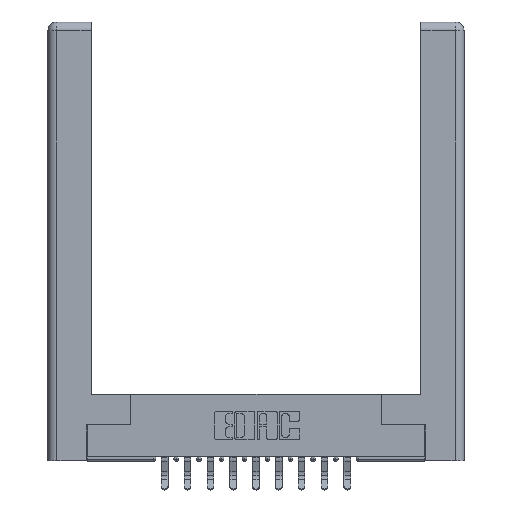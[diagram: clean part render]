
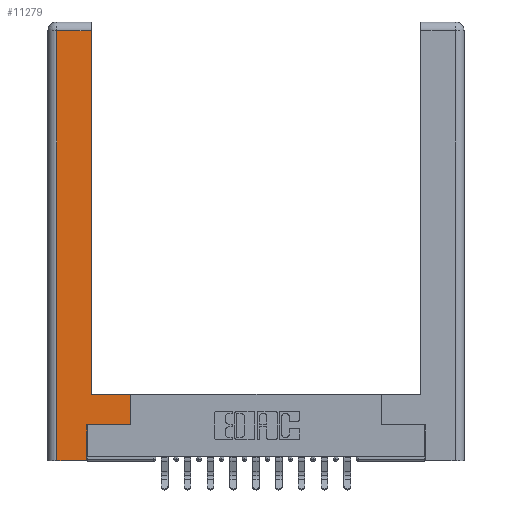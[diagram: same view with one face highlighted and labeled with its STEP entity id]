
A CAD part, top view. The second image highlights one B-rep face of the part: STEP entity #11279.
In plain terms, the highlighted planar face has unit normal (0, 0, 1).
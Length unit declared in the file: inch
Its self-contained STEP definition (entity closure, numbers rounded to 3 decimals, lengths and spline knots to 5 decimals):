
#179 = AXIS2_PLACEMENT_3D ( 'NONE', #3150, #12336, #1984 ) ;
#223 = VERTEX_POINT ( 'NONE', #7931 ) ;
#226 = LINE ( 'NONE', #12512, #13695 ) ;
#437 = ORIENTED_EDGE ( 'NONE', *, *, #2153, .T. ) ;
#646 = VECTOR ( 'NONE', #8179, 39.37008 ) ;
#1049 = ORIENTED_EDGE ( 'NONE', *, *, #10525, .T. ) ;
#1099 = EDGE_CURVE ( 'NONE', #14840, #5344, #5304, .T. ) ;
#1471 = CARTESIAN_POINT ( 'NONE',  ( 0.0615, 2.94, 0. ) ) ;
#1791 = ORIENTED_EDGE ( 'NONE', *, *, #7333, .T. ) ;
#1884 = VECTOR ( 'NONE', #2196, 39.37008 ) ;
#1984 = DIRECTION ( 'NONE',  ( -1., 0., 0. ) ) ;
#2096 = LINE ( 'NONE', #7029, #12366 ) ;
#2153 = EDGE_CURVE ( 'NONE', #2944, #7525, #11709, .T. ) ;
#2196 = DIRECTION ( 'NONE',  ( 1., 0., 0. ) ) ;
#2628 = DIRECTION ( 'NONE',  ( 1., 0., 0. ) ) ;
#2869 = ORIENTED_EDGE ( 'NONE', *, *, #2991, .T. ) ;
#2944 = VERTEX_POINT ( 'NONE', #7963 ) ;
#2991 = EDGE_CURVE ( 'NONE', #14811, #223, #11489, .T. ) ;
#3150 = CARTESIAN_POINT ( 'NONE',  ( 0., 0., 0. ) ) ;
#3233 = LINE ( 'NONE', #11799, #10904 ) ;
#3268 = FACE_OUTER_BOUND ( 'NONE', #3476, .T. ) ;
#3476 = EDGE_LOOP ( 'NONE', ( #2869, #1791, #5058, #13850, #15100, #437, #6059, #1049 ) ) ;
#3784 = CARTESIAN_POINT ( 'NONE',  ( 0.0615, 2.94, 0. ) ) ;
#4570 = CARTESIAN_POINT ( 'NONE',  ( 0.0615, 0., 0. ) ) ;
#4951 = EDGE_CURVE ( 'NONE', #5344, #2944, #2096, .T. ) ;
#5058 = ORIENTED_EDGE ( 'NONE', *, *, #6686, .T. ) ;
#5106 = CARTESIAN_POINT ( 'NONE',  ( 0.565, 0.245, 0. ) ) ;
#5128 = CARTESIAN_POINT ( 'NONE',  ( 0.265, 0., 0. ) ) ;
#5304 = LINE ( 'NONE', #9996, #1884 ) ;
#5344 = VERTEX_POINT ( 'NONE', #5128 ) ;
#5439 = CARTESIAN_POINT ( 'NONE',  ( 0.295, 3., 0. ) ) ;
#5658 = DIRECTION ( 'NONE',  ( 0., -1., 0. ) ) ;
#6059 = ORIENTED_EDGE ( 'NONE', *, *, #6863, .T. ) ;
#6686 = EDGE_CURVE ( 'NONE', #16604, #14840, #3233, .T. ) ;
#6863 = EDGE_CURVE ( 'NONE', #7525, #11368, #226, .T. ) ;
#7029 = CARTESIAN_POINT ( 'NONE',  ( 0.265, 0.245, 0. ) ) ;
#7333 = EDGE_CURVE ( 'NONE', #223, #16604, #10656, .T. ) ;
#7525 = VERTEX_POINT ( 'NONE', #16561 ) ;
#7920 = VECTOR ( 'NONE', #13492, 39.37008 ) ;
#7931 = CARTESIAN_POINT ( 'NONE',  ( 0.295, 2.94, 0. ) ) ;
#7963 = CARTESIAN_POINT ( 'NONE',  ( 0.265, 0.245, 0. ) ) ;
#8179 = DIRECTION ( 'NONE',  ( 0., 1., 0. ) ) ;
#8254 = DIRECTION ( 'NONE',  ( -1., 0., 0. ) ) ;
#8311 = DIRECTION ( 'NONE',  ( 0., 1., 0. ) ) ;
#8440 = VECTOR ( 'NONE', #8254, 39.37008 ) ;
#9734 = LINE ( 'NONE', #10722, #7920 ) ;
#9996 = CARTESIAN_POINT ( 'NONE',  ( 0.265, 0., 0. ) ) ;
#10525 = EDGE_CURVE ( 'NONE', #11368, #14811, #9734, .T. ) ;
#10656 = LINE ( 'NONE', #1471, #8440 ) ;
#10722 = CARTESIAN_POINT ( 'NONE',  ( 0.295, 0.45, 0. ) ) ;
#10821 = PLANE ( 'NONE',  #179 ) ;
#10904 = VECTOR ( 'NONE', #5658, 39.37008 ) ;
#11279 = ADVANCED_FACE ( 'NONE', ( #3268 ), #10821, .F. ) ;
#11368 = VERTEX_POINT ( 'NONE', #11590 ) ;
#11489 = LINE ( 'NONE', #5439, #646 ) ;
#11590 = CARTESIAN_POINT ( 'NONE',  ( 0.565, 0.45, 0. ) ) ;
#11709 = LINE ( 'NONE', #5106, #14107 ) ;
#11799 = CARTESIAN_POINT ( 'NONE',  ( 0.0615, 0., 0. ) ) ;
#12336 = DIRECTION ( 'NONE',  ( 0., 0., -1. ) ) ;
#12366 = VECTOR ( 'NONE', #8311, 39.37008 ) ;
#12512 = CARTESIAN_POINT ( 'NONE',  ( 0.565, 0.45, 0. ) ) ;
#13492 = DIRECTION ( 'NONE',  ( -1., 0., 0. ) ) ;
#13695 = VECTOR ( 'NONE', #15152, 39.37008 ) ;
#13850 = ORIENTED_EDGE ( 'NONE', *, *, #1099, .T. ) ;
#14107 = VECTOR ( 'NONE', #2628, 39.37008 ) ;
#14811 = VERTEX_POINT ( 'NONE', #16100 ) ;
#14840 = VERTEX_POINT ( 'NONE', #4570 ) ;
#15100 = ORIENTED_EDGE ( 'NONE', *, *, #4951, .T. ) ;
#15152 = DIRECTION ( 'NONE',  ( 0., 1., 0. ) ) ;
#16100 = CARTESIAN_POINT ( 'NONE',  ( 0.295, 0.45, 0. ) ) ;
#16561 = CARTESIAN_POINT ( 'NONE',  ( 0.565, 0.245, 0. ) ) ;
#16604 = VERTEX_POINT ( 'NONE', #3784 ) ;
